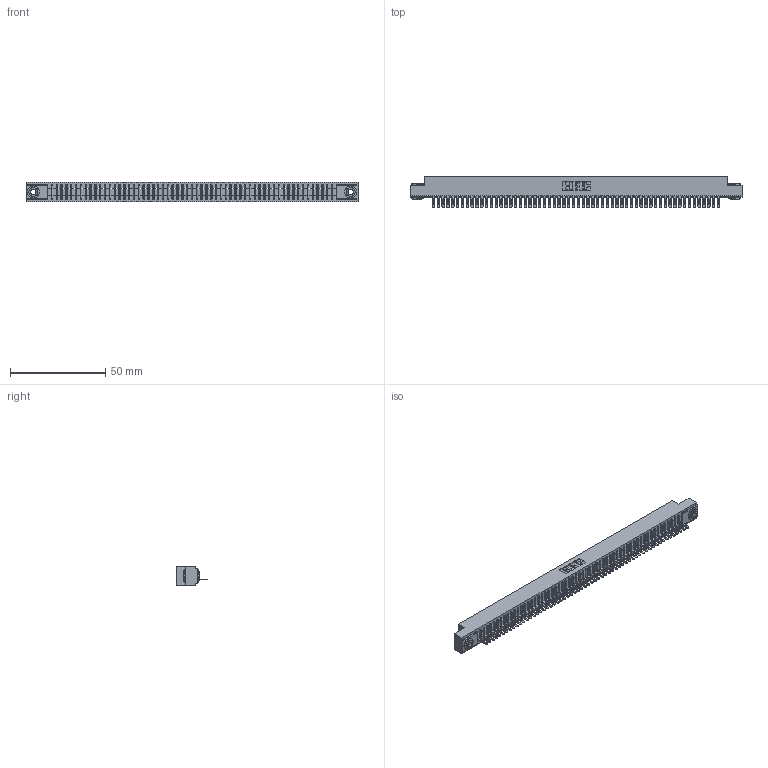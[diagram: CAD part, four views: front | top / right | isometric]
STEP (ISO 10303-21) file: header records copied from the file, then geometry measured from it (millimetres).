
FILE_DESCRIPTION (( 'STEP AP203' ), '1' );
FILE_NAME ('341-060-500-103.STEP', '2018-08-07T16:59:41', ( '' ), ( '' ), 'SwSTEP 2.0', 'SolidWorks 2016', '' );
FILE_SCHEMA (( 'CONFIG_CONTROL_DESIGN' ));
Length unit declared in the file: inch
Products named in the file (4): 345-250-002_345-250-002-102; 341-060-500-103; 341 Part_.156 (3.96) Dia Mounting Holes; 341-292-001_341-292-100
Assembly tree (63 placements, depth 2):
  341-060-500-103
    341 Part_.156 (3.96) Dia Mounting Holes
    341-292-001_341-292-100  x60
    345-250-002_345-250-002-102  x2
Bounding box: 174.62 x 16.69 x 10.16 mm (x, y, z)
Volume: 12560.5 mm3; surface area: 20621.5 mm2
Topology: 63 solids, 63 shells, 5088 faces, 14648 edges, 9398 vertices
Faces by surface type: plane 3032, cylinder 1808, sphere 122, torus 118, cone 8
Entity records: 69368 total; most frequent: CARTESIAN_POINT 11769, ORIENTED_EDGE 11748, DIRECTION 11366, EDGE_CURVE 5874, LINE 4752, VECTOR 4752, VERTEX_POINT 3710, AXIS2_PLACEMENT_3D 3307
